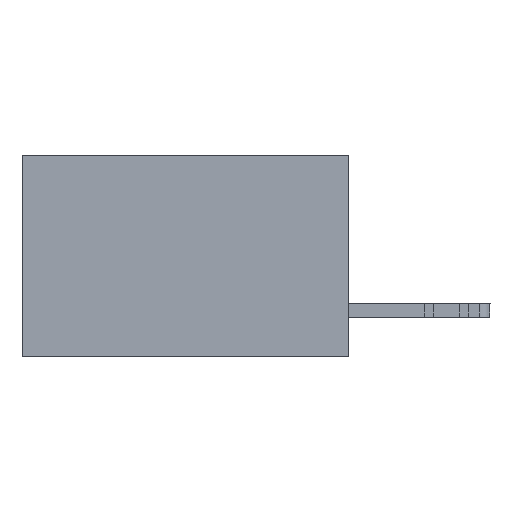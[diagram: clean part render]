
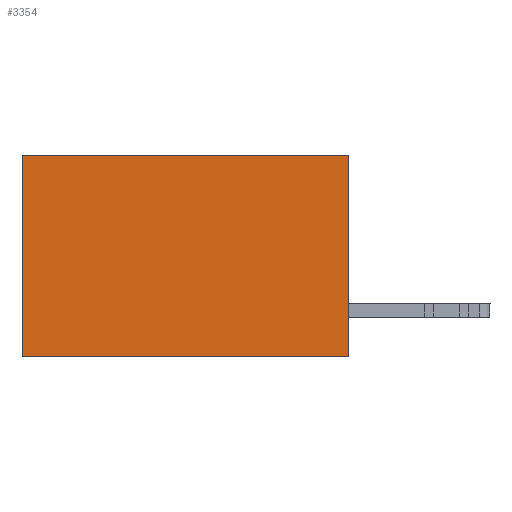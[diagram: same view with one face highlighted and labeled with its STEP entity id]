
A CAD part, left-side view. The second image highlights one B-rep face of the part: STEP entity #3354.
In plain terms, the highlighted planar face has unit normal (-1, 0, 0).
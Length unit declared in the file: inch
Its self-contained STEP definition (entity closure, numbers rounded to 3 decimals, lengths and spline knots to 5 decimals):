
#94 = ORIENTED_EDGE ( 'NONE', *, *, #9389, .F. ) ;
#1089 = CARTESIAN_POINT ( 'NONE',  ( 0.298, 0., 0. ) ) ;
#1302 = DIRECTION ( 'NONE',  ( 0., 0., -1. ) ) ;
#2650 = VERTEX_POINT ( 'NONE', #23418 ) ;
#3354 = ADVANCED_FACE ( 'NONE', ( #14048 ), #17383, .F. ) ;
#5836 = VECTOR ( 'NONE', #8735, 39.37008 ) ;
#5957 = CARTESIAN_POINT ( 'NONE',  ( 0.298, 0., 0. ) ) ;
#6029 = EDGE_LOOP ( 'NONE', ( #9240, #21727, #94, #27386 ) ) ;
#6580 = LINE ( 'NONE', #21567, #5836 ) ;
#7729 = LINE ( 'NONE', #13127, #23051 ) ;
#7897 = DIRECTION ( 'NONE',  ( 1., 0., 0. ) ) ;
#8735 = DIRECTION ( 'NONE',  ( 0., 0., -1. ) ) ;
#9240 = ORIENTED_EDGE ( 'NONE', *, *, #20409, .T. ) ;
#9354 = EDGE_CURVE ( 'NONE', #27437, #2650, #7729, .T. ) ;
#9389 = EDGE_CURVE ( 'NONE', #27437, #19909, #25308, .T. ) ;
#11980 = CARTESIAN_POINT ( 'NONE',  ( 0.298, 0., 0. ) ) ;
#12161 = VECTOR ( 'NONE', #21912, 39.37008 ) ;
#13127 = CARTESIAN_POINT ( 'NONE',  ( 0.298, 0., 0. ) ) ;
#14048 = FACE_OUTER_BOUND ( 'NONE', #6029, .T. ) ;
#16675 = VECTOR ( 'NONE', #1302, 39.37008 ) ;
#16872 = CARTESIAN_POINT ( 'NONE',  ( 0.298, 0., -0.37 ) ) ;
#16916 = VERTEX_POINT ( 'NONE', #30572 ) ;
#17383 = PLANE ( 'NONE',  #29152 ) ;
#17603 = DIRECTION ( 'NONE',  ( 0., 0., -1. ) ) ;
#17828 = DIRECTION ( 'NONE',  ( 0., 1., 0. ) ) ;
#19909 = VERTEX_POINT ( 'NONE', #28387 ) ;
#19974 = EDGE_CURVE ( 'NONE', #19909, #16916, #21897, .T. ) ;
#20409 = EDGE_CURVE ( 'NONE', #2650, #16916, #6580, .T. ) ;
#21567 = CARTESIAN_POINT ( 'NONE',  ( 0.298, 0.6, 0. ) ) ;
#21727 = ORIENTED_EDGE ( 'NONE', *, *, #19974, .F. ) ;
#21897 = LINE ( 'NONE', #16872, #12161 ) ;
#21912 = DIRECTION ( 'NONE',  ( 0., 1., 0. ) ) ;
#23051 = VECTOR ( 'NONE', #17828, 39.37008 ) ;
#23418 = CARTESIAN_POINT ( 'NONE',  ( 0.298, 0.6, 0. ) ) ;
#25308 = LINE ( 'NONE', #5957, #16675 ) ;
#27386 = ORIENTED_EDGE ( 'NONE', *, *, #9354, .T. ) ;
#27437 = VERTEX_POINT ( 'NONE', #11980 ) ;
#28387 = CARTESIAN_POINT ( 'NONE',  ( 0.298, 0., -0.37 ) ) ;
#29152 = AXIS2_PLACEMENT_3D ( 'NONE', #1089, #7897, #17603 ) ;
#30572 = CARTESIAN_POINT ( 'NONE',  ( 0.298, 0.6, -0.37 ) ) ;
